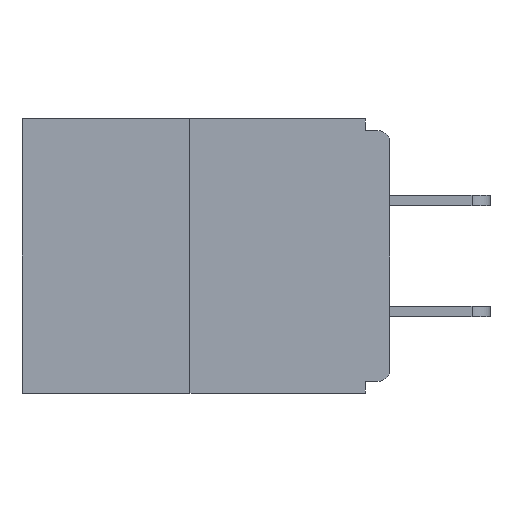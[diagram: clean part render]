
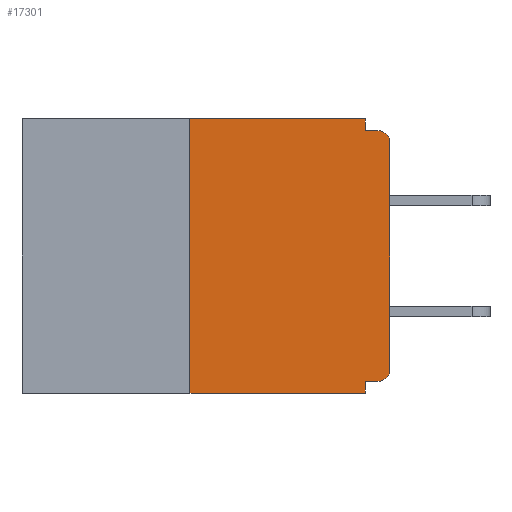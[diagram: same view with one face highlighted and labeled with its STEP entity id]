
A CAD part, left-side view. The second image highlights one B-rep face of the part: STEP entity #17301.
In plain terms, the highlighted planar face has unit normal (-1, 0, 0).
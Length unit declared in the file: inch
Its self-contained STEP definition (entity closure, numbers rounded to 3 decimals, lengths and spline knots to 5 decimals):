
#257 = CARTESIAN_POINT ( 'NONE',  ( 0., 0.25, 0. ) ) ;
#1359 = DIRECTION ( 'NONE',  ( 0., 0., -1. ) ) ;
#1515 = VECTOR ( 'NONE', #19342, 39.37008 ) ;
#1569 = VERTEX_POINT ( 'NONE', #5865 ) ;
#1736 = VECTOR ( 'NONE', #21321, 39.37008 ) ;
#2226 = ORIENTED_EDGE ( 'NONE', *, *, #12903, .F. ) ;
#2608 = EDGE_CURVE ( 'NONE', #15697, #22060, #6198, .T. ) ;
#2899 = ORIENTED_EDGE ( 'NONE', *, *, #6354, .T. ) ;
#3598 = AXIS2_PLACEMENT_3D ( 'NONE', #17314, #10127, #15373 ) ;
#3660 = DIRECTION ( 'NONE',  ( 0., 1., 0. ) ) ;
#3960 = LINE ( 'NONE', #15800, #1736 ) ;
#4141 = VERTEX_POINT ( 'NONE', #8368 ) ;
#4312 = VERTEX_POINT ( 'NONE', #4426 ) ;
#4426 = CARTESIAN_POINT ( 'NONE',  ( 0., 0., -0.313 ) ) ;
#4883 = CARTESIAN_POINT ( 'NONE',  ( 0., 0.015, -0.313 ) ) ;
#5096 = FACE_OUTER_BOUND ( 'NONE', #18538, .T. ) ;
#5340 = CARTESIAN_POINT ( 'NONE',  ( 0., 0.031, -0.343 ) ) ;
#5865 = CARTESIAN_POINT ( 'NONE',  ( 0., 0.015, -0.328 ) ) ;
#5930 = ORIENTED_EDGE ( 'NONE', *, *, #9429, .F. ) ;
#6198 = LINE ( 'NONE', #10764, #1515 ) ;
#6283 = DIRECTION ( 'NONE',  ( -1., 0., 0. ) ) ;
#6354 = EDGE_CURVE ( 'NONE', #4312, #17006, #3960, .T. ) ;
#6360 = DIRECTION ( 'NONE',  ( 0., 0., -1. ) ) ;
#6380 = VECTOR ( 'NONE', #16416, 39.37008 ) ;
#6561 = CARTESIAN_POINT ( 'NONE',  ( 0., 0.031, -0.015 ) ) ;
#7738 = AXIS2_PLACEMENT_3D ( 'NONE', #4883, #22365, #1359 ) ;
#7814 = ORIENTED_EDGE ( 'NONE', *, *, #12039, .F. ) ;
#8039 = LINE ( 'NONE', #257, #10789 ) ;
#8225 = EDGE_CURVE ( 'NONE', #15697, #12177, #8039, .T. ) ;
#8368 = CARTESIAN_POINT ( 'NONE',  ( 0., 0.031, 0. ) ) ;
#8494 = LINE ( 'NONE', #17130, #10960 ) ;
#9429 = EDGE_CURVE ( 'NONE', #1569, #10501, #10188, .T. ) ;
#9519 = VECTOR ( 'NONE', #10239, 39.37008 ) ;
#10032 = DIRECTION ( 'NONE',  ( 0., -1., 0. ) ) ;
#10127 = DIRECTION ( 'NONE',  ( 1., 0., 0. ) ) ;
#10149 = EDGE_CURVE ( 'NONE', #17006, #11246, #17307, .T. ) ;
#10188 = LINE ( 'NONE', #19587, #12364 ) ;
#10239 = DIRECTION ( 'NONE',  ( 0., -1., 0. ) ) ;
#10268 = CARTESIAN_POINT ( 'NONE',  ( 0., 0.031, 0. ) ) ;
#10501 = VERTEX_POINT ( 'NONE', #21417 ) ;
#10764 = CARTESIAN_POINT ( 'NONE',  ( 0., 0.46, -0.343 ) ) ;
#10789 = VECTOR ( 'NONE', #14014, 39.37008 ) ;
#10960 = VECTOR ( 'NONE', #10032, 39.37008 ) ;
#11246 = VERTEX_POINT ( 'NONE', #14143 ) ;
#11594 = CARTESIAN_POINT ( 'NONE',  ( 0., 0.25, -0.343 ) ) ;
#11669 = ORIENTED_EDGE ( 'NONE', *, *, #10149, .T. ) ;
#12039 = EDGE_CURVE ( 'NONE', #12177, #4141, #15243, .T. ) ;
#12073 = ORIENTED_EDGE ( 'NONE', *, *, #2608, .T. ) ;
#12177 = VERTEX_POINT ( 'NONE', #14310 ) ;
#12364 = VECTOR ( 'NONE', #3660, 39.37008 ) ;
#12683 = LINE ( 'NONE', #10268, #13757 ) ;
#12747 = DIRECTION ( 'NONE',  ( 0., 0., -1. ) ) ;
#12903 = EDGE_CURVE ( 'NONE', #10501, #22060, #18711, .T. ) ;
#13757 = VECTOR ( 'NONE', #12747, 39.37008 ) ;
#14014 = DIRECTION ( 'NONE',  ( 0., 0., 1. ) ) ;
#14143 = CARTESIAN_POINT ( 'NONE',  ( 0., 0.015, -0.015 ) ) ;
#14310 = CARTESIAN_POINT ( 'NONE',  ( 0., 0.25, 0. ) ) ;
#15046 = CARTESIAN_POINT ( 'NONE',  ( 0., 0.015, -0.03 ) ) ;
#15103 = EDGE_CURVE ( 'NONE', #16629, #11246, #8494, .T. ) ;
#15243 = LINE ( 'NONE', #19038, #9519 ) ;
#15373 = DIRECTION ( 'NONE',  ( 0., 0., -1. ) ) ;
#15452 = ORIENTED_EDGE ( 'NONE', *, *, #15103, .F. ) ;
#15601 = AXIS2_PLACEMENT_3D ( 'NONE', #15046, #6283, #6360 ) ;
#15697 = VERTEX_POINT ( 'NONE', #11594 ) ;
#15800 = CARTESIAN_POINT ( 'NONE',  ( 0., 0., 0. ) ) ;
#16416 = DIRECTION ( 'NONE',  ( 0., 0., -1. ) ) ;
#16629 = VERTEX_POINT ( 'NONE', #6561 ) ;
#16687 = CARTESIAN_POINT ( 'NONE',  ( 0., 0., -0.03 ) ) ;
#17006 = VERTEX_POINT ( 'NONE', #16687 ) ;
#17130 = CARTESIAN_POINT ( 'NONE',  ( 0., 0., -0.015 ) ) ;
#17301 = ADVANCED_FACE ( 'NONE', ( #5096 ), #22374, .F. ) ;
#17307 = CIRCLE ( 'NONE', #15601, 0.015 ) ;
#17314 = CARTESIAN_POINT ( 'NONE',  ( 0., 0.46, 0. ) ) ;
#18460 = ORIENTED_EDGE ( 'NONE', *, *, #18563, .T. ) ;
#18538 = EDGE_LOOP ( 'NONE', ( #7814, #21015, #12073, #2226, #5930, #18460, #2899, #11669, #15452, #21958 ) ) ;
#18563 = EDGE_CURVE ( 'NONE', #1569, #4312, #22031, .T. ) ;
#18603 = EDGE_CURVE ( 'NONE', #4141, #16629, #12683, .T. ) ;
#18711 = LINE ( 'NONE', #20190, #6380 ) ;
#19038 = CARTESIAN_POINT ( 'NONE',  ( 0., 0.46, 0. ) ) ;
#19342 = DIRECTION ( 'NONE',  ( 0., -1., 0. ) ) ;
#19587 = CARTESIAN_POINT ( 'NONE',  ( 0., 0., -0.328 ) ) ;
#20190 = CARTESIAN_POINT ( 'NONE',  ( 0., 0.031, -0.343 ) ) ;
#21015 = ORIENTED_EDGE ( 'NONE', *, *, #8225, .F. ) ;
#21321 = DIRECTION ( 'NONE',  ( 0., 0., 1. ) ) ;
#21417 = CARTESIAN_POINT ( 'NONE',  ( 0., 0.031, -0.328 ) ) ;
#21958 = ORIENTED_EDGE ( 'NONE', *, *, #18603, .F. ) ;
#22031 = CIRCLE ( 'NONE', #7738, 0.015 ) ;
#22060 = VERTEX_POINT ( 'NONE', #5340 ) ;
#22365 = DIRECTION ( 'NONE',  ( -1., 0., 0. ) ) ;
#22374 = PLANE ( 'NONE',  #3598 ) ;
